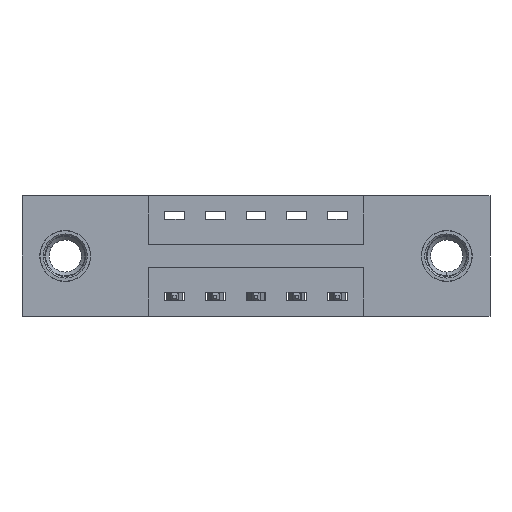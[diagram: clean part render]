
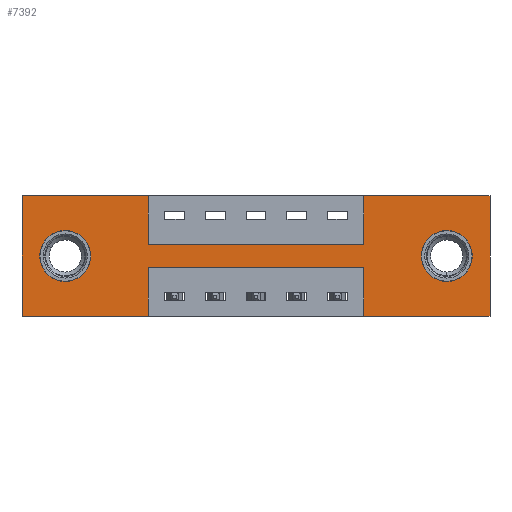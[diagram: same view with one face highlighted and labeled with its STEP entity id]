
A CAD part, front view. The second image highlights one B-rep face of the part: STEP entity #7392.
In plain terms, the highlighted planar face has unit normal (0, -1, 0).
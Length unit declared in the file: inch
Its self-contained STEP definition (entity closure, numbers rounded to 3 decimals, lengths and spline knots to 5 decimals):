
#20 = DIRECTION ( 'NONE',  ( 0., 0., 1. ) ) ;
#57 = ORIENTED_EDGE ( 'NONE', *, *, #3315, .F. ) ;
#130 = CIRCLE ( 'NONE', #2872, 0.078 ) ;
#160 = LINE ( 'NONE', #5250, #5417 ) ;
#232 = ORIENTED_EDGE ( 'NONE', *, *, #2372, .F. ) ;
#260 = AXIS2_PLACEMENT_3D ( 'NONE', #4169, #2738, #9108 ) ;
#290 = CIRCLE ( 'NONE', #885, 0.078 ) ;
#315 = EDGE_LOOP ( 'NONE', ( #1232, #4081 ) ) ;
#338 = EDGE_LOOP ( 'NONE', ( #57, #5037, #9048, #232, #4255, #5353, #2840, #2777, #7854, #4638, #5002, #3883 ) ) ;
#447 = VERTEX_POINT ( 'NONE', #6313 ) ;
#527 = FACE_BOUND ( 'NONE', #315, .T. ) ;
#534 = DIRECTION ( 'NONE',  ( -1., 0., 0. ) ) ;
#580 = DIRECTION ( 'NONE',  ( 0., 0., 1. ) ) ;
#617 = CARTESIAN_POINT ( 'NONE',  ( 0., 0., -0.37 ) ) ;
#644 = VERTEX_POINT ( 'NONE', #3879 ) ;
#663 = FACE_OUTER_BOUND ( 'NONE', #338, .T. ) ;
#858 = EDGE_CURVE ( 'NONE', #963, #6330, #290, .T. ) ;
#873 = CARTESIAN_POINT ( 'NONE',  ( 0., 0., 0. ) ) ;
#885 = AXIS2_PLACEMENT_3D ( 'NONE', #1720, #5476, #4600 ) ;
#963 = VERTEX_POINT ( 'NONE', #1515 ) ;
#1232 = ORIENTED_EDGE ( 'NONE', *, *, #858, .T. ) ;
#1426 = EDGE_CURVE ( 'NONE', #2074, #8052, #6273, .T. ) ;
#1506 = AXIS2_PLACEMENT_3D ( 'NONE', #3690, #5053, #5664 ) ;
#1515 = CARTESIAN_POINT ( 'NONE',  ( 0.1325, 0., -0.107 ) ) ;
#1522 = CARTESIAN_POINT ( 'NONE',  ( 0., 0., -0.37 ) ) ;
#1545 = VECTOR ( 'NONE', #5526, 39.37008 ) ;
#1549 = LINE ( 'NONE', #7316, #5166 ) ;
#1720 = CARTESIAN_POINT ( 'NONE',  ( 0.1325, 0., -0.185 ) ) ;
#1739 = VERTEX_POINT ( 'NONE', #8214 ) ;
#1925 = DIRECTION ( 'NONE',  ( 0., 1., 0. ) ) ;
#1938 = CARTESIAN_POINT ( 'NONE',  ( 1.435, 0., 0. ) ) ;
#2017 = EDGE_CURVE ( 'NONE', #8052, #6205, #5270, .T. ) ;
#2032 = DIRECTION ( 'NONE',  ( 1., 0., 0. ) ) ;
#2059 = VERTEX_POINT ( 'NONE', #1938 ) ;
#2074 = VERTEX_POINT ( 'NONE', #9276 ) ;
#2086 = EDGE_CURVE ( 'NONE', #6330, #963, #5707, .T. ) ;
#2312 = EDGE_CURVE ( 'NONE', #1739, #4106, #160, .T. ) ;
#2362 = CARTESIAN_POINT ( 'NONE',  ( 1.0475, 0., -0.15 ) ) ;
#2372 = EDGE_CURVE ( 'NONE', #7878, #2074, #5922, .T. ) ;
#2535 = VERTEX_POINT ( 'NONE', #7340 ) ;
#2610 = VERTEX_POINT ( 'NONE', #1522 ) ;
#2611 = LINE ( 'NONE', #7464, #7718 ) ;
#2712 = LINE ( 'NONE', #2803, #2755 ) ;
#2738 = DIRECTION ( 'NONE',  ( 0., 1., 0. ) ) ;
#2755 = VECTOR ( 'NONE', #9311, 39.37008 ) ;
#2777 = ORIENTED_EDGE ( 'NONE', *, *, #2312, .F. ) ;
#2783 = CARTESIAN_POINT ( 'NONE',  ( 1.435, 0., -0.37 ) ) ;
#2803 = CARTESIAN_POINT ( 'NONE',  ( 0.3875, 0., -0.37 ) ) ;
#2840 = ORIENTED_EDGE ( 'NONE', *, *, #6087, .F. ) ;
#2872 = AXIS2_PLACEMENT_3D ( 'NONE', #3882, #1925, #6833 ) ;
#2883 = CARTESIAN_POINT ( 'NONE',  ( 1.0475, 0., 0. ) ) ;
#2935 = EDGE_CURVE ( 'NONE', #2059, #7878, #2611, .T. ) ;
#3023 = VECTOR ( 'NONE', #3892, 39.37008 ) ;
#3103 = DIRECTION ( 'NONE',  ( 1., 0., 0. ) ) ;
#3179 = AXIS2_PLACEMENT_3D ( 'NONE', #617, #4826, #3422 ) ;
#3315 = EDGE_CURVE ( 'NONE', #6205, #7060, #2712, .T. ) ;
#3422 = DIRECTION ( 'NONE',  ( 0., 0., -1. ) ) ;
#3490 = DIRECTION ( 'NONE',  ( 0., 0., -1. ) ) ;
#3505 = FACE_BOUND ( 'NONE', #8406, .T. ) ;
#3599 = VECTOR ( 'NONE', #3490, 39.37008 ) ;
#3690 = CARTESIAN_POINT ( 'NONE',  ( 0.1325, 0., -0.185 ) ) ;
#3703 = DIRECTION ( 'NONE',  ( 1., 0., 0. ) ) ;
#3879 = CARTESIAN_POINT ( 'NONE',  ( 1.3025, 0., -0.263 ) ) ;
#3882 = CARTESIAN_POINT ( 'NONE',  ( 1.3025, 0., -0.185 ) ) ;
#3883 = ORIENTED_EDGE ( 'NONE', *, *, #3969, .F. ) ;
#3892 = DIRECTION ( 'NONE',  ( -1., 0., 0. ) ) ;
#3969 = EDGE_CURVE ( 'NONE', #7060, #2610, #8310, .T. ) ;
#4081 = ORIENTED_EDGE ( 'NONE', *, *, #2086, .T. ) ;
#4106 = VERTEX_POINT ( 'NONE', #2362 ) ;
#4159 = CARTESIAN_POINT ( 'NONE',  ( 1.0475, 0., -0.37 ) ) ;
#4169 = CARTESIAN_POINT ( 'NONE',  ( 1.3025, 0., -0.185 ) ) ;
#4255 = ORIENTED_EDGE ( 'NONE', *, *, #2935, .F. ) ;
#4600 = DIRECTION ( 'NONE',  ( 0., 0., 1. ) ) ;
#4638 = ORIENTED_EDGE ( 'NONE', *, *, #5747, .F. ) ;
#4639 = VECTOR ( 'NONE', #2032, 39.37008 ) ;
#4721 = CARTESIAN_POINT ( 'NONE',  ( 0., 0., -0.37 ) ) ;
#4826 = DIRECTION ( 'NONE',  ( 0., -1., 0. ) ) ;
#4928 = LINE ( 'NONE', #2883, #8254 ) ;
#4935 = CIRCLE ( 'NONE', #260, 0.078 ) ;
#4998 = PLANE ( 'NONE',  #3179 ) ;
#5002 = ORIENTED_EDGE ( 'NONE', *, *, #8432, .F. ) ;
#5037 = ORIENTED_EDGE ( 'NONE', *, *, #2017, .F. ) ;
#5053 = DIRECTION ( 'NONE',  ( 0., 1., 0. ) ) ;
#5087 = LINE ( 'NONE', #8573, #3599 ) ;
#5166 = VECTOR ( 'NONE', #3703, 39.37008 ) ;
#5226 = EDGE_CURVE ( 'NONE', #6648, #2059, #1549, .T. ) ;
#5250 = CARTESIAN_POINT ( 'NONE',  ( 0.3875, 0., -0.15 ) ) ;
#5270 = LINE ( 'NONE', #6895, #3023 ) ;
#5353 = ORIENTED_EDGE ( 'NONE', *, *, #5226, .F. ) ;
#5417 = VECTOR ( 'NONE', #3103, 39.37008 ) ;
#5476 = DIRECTION ( 'NONE',  ( 0., 1., 0. ) ) ;
#5526 = DIRECTION ( 'NONE',  ( -1., 0., 0. ) ) ;
#5590 = LINE ( 'NONE', #8463, #4639 ) ;
#5652 = VECTOR ( 'NONE', #20, 39.37008 ) ;
#5659 = CARTESIAN_POINT ( 'NONE',  ( 0.3875, 0., -0.22 ) ) ;
#5664 = DIRECTION ( 'NONE',  ( 0., 0., 1. ) ) ;
#5707 = CIRCLE ( 'NONE', #1506, 0.078 ) ;
#5747 = EDGE_CURVE ( 'NONE', #447, #2535, #5590, .T. ) ;
#5865 = CARTESIAN_POINT ( 'NONE',  ( 1.0475, 0., -0.22 ) ) ;
#5922 = LINE ( 'NONE', #7015, #7869 ) ;
#6087 = EDGE_CURVE ( 'NONE', #4106, #6648, #4928, .T. ) ;
#6205 = VERTEX_POINT ( 'NONE', #5659 ) ;
#6273 = LINE ( 'NONE', #4159, #7381 ) ;
#6313 = CARTESIAN_POINT ( 'NONE',  ( 0., 0., 0. ) ) ;
#6330 = VERTEX_POINT ( 'NONE', #6444 ) ;
#6430 = EDGE_CURVE ( 'NONE', #8314, #644, #4935, .T. ) ;
#6444 = CARTESIAN_POINT ( 'NONE',  ( 0.1325, 0., -0.263 ) ) ;
#6561 = ORIENTED_EDGE ( 'NONE', *, *, #6430, .T. ) ;
#6648 = VERTEX_POINT ( 'NONE', #7239 ) ;
#6833 = DIRECTION ( 'NONE',  ( 0., 0., -1. ) ) ;
#6895 = CARTESIAN_POINT ( 'NONE',  ( 0.3875, 0., -0.22 ) ) ;
#7015 = CARTESIAN_POINT ( 'NONE',  ( 0., 0., -0.37 ) ) ;
#7060 = VERTEX_POINT ( 'NONE', #7374 ) ;
#7138 = EDGE_CURVE ( 'NONE', #644, #8314, #130, .T. ) ;
#7239 = CARTESIAN_POINT ( 'NONE',  ( 1.0475, 0., 0. ) ) ;
#7316 = CARTESIAN_POINT ( 'NONE',  ( 0., 0., 0. ) ) ;
#7340 = CARTESIAN_POINT ( 'NONE',  ( 0.3875, 0., 0. ) ) ;
#7374 = CARTESIAN_POINT ( 'NONE',  ( 0.3875, 0., -0.37 ) ) ;
#7381 = VECTOR ( 'NONE', #580, 39.37008 ) ;
#7392 = ADVANCED_FACE ( 'NONE', ( #3505, #527, #663 ), #4998, .T. ) ;
#7464 = CARTESIAN_POINT ( 'NONE',  ( 1.435, 0., 0. ) ) ;
#7718 = VECTOR ( 'NONE', #9023, 39.37008 ) ;
#7751 = EDGE_CURVE ( 'NONE', #2535, #1739, #5087, .T. ) ;
#7854 = ORIENTED_EDGE ( 'NONE', *, *, #7751, .F. ) ;
#7869 = VECTOR ( 'NONE', #534, 39.37008 ) ;
#7878 = VERTEX_POINT ( 'NONE', #2783 ) ;
#8007 = ORIENTED_EDGE ( 'NONE', *, *, #7138, .T. ) ;
#8052 = VERTEX_POINT ( 'NONE', #5865 ) ;
#8214 = CARTESIAN_POINT ( 'NONE',  ( 0.3875, 0., -0.15 ) ) ;
#8254 = VECTOR ( 'NONE', #8512, 39.37008 ) ;
#8310 = LINE ( 'NONE', #4721, #1545 ) ;
#8314 = VERTEX_POINT ( 'NONE', #8469 ) ;
#8406 = EDGE_LOOP ( 'NONE', ( #6561, #8007 ) ) ;
#8432 = EDGE_CURVE ( 'NONE', #2610, #447, #8609, .T. ) ;
#8463 = CARTESIAN_POINT ( 'NONE',  ( 0., 0., 0. ) ) ;
#8469 = CARTESIAN_POINT ( 'NONE',  ( 1.3025, 0., -0.107 ) ) ;
#8512 = DIRECTION ( 'NONE',  ( 0., 0., 1. ) ) ;
#8573 = CARTESIAN_POINT ( 'NONE',  ( 0.3875, 0., 0. ) ) ;
#8609 = LINE ( 'NONE', #873, #5652 ) ;
#9023 = DIRECTION ( 'NONE',  ( 0., 0., -1. ) ) ;
#9048 = ORIENTED_EDGE ( 'NONE', *, *, #1426, .F. ) ;
#9108 = DIRECTION ( 'NONE',  ( 0., 0., -1. ) ) ;
#9276 = CARTESIAN_POINT ( 'NONE',  ( 1.0475, 0., -0.37 ) ) ;
#9311 = DIRECTION ( 'NONE',  ( 0., 0., -1. ) ) ;
